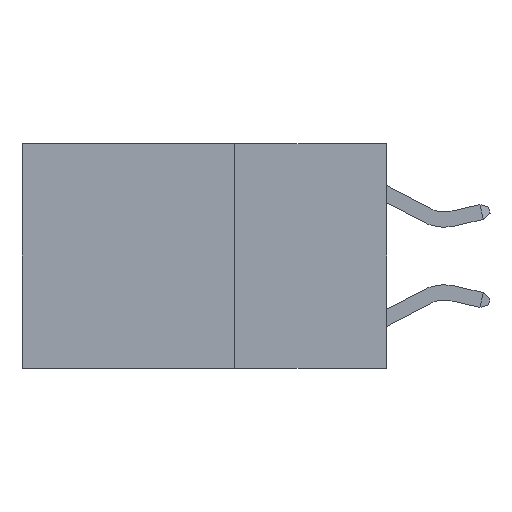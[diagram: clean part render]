
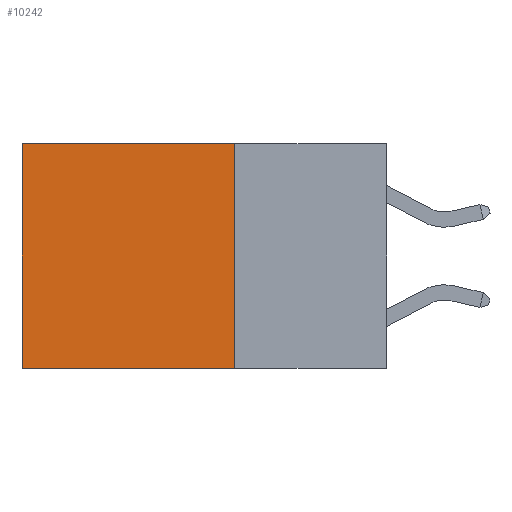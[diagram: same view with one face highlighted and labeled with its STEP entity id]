
A CAD part, left-side view. The second image highlights one B-rep face of the part: STEP entity #10242.
In plain terms, the highlighted planar face has unit normal (-1, 0, 0).
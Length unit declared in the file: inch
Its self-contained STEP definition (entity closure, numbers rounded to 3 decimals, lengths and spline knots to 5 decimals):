
#356 = DIRECTION ( 'NONE',  ( 0., 0., -1. ) ) ;
#781 = CARTESIAN_POINT ( 'NONE',  ( 0.2625, 0.25, -0.37 ) ) ;
#1396 = AXIS2_PLACEMENT_3D ( 'NONE', #16977, #13441, #356 ) ;
#1850 = LINE ( 'NONE', #19306, #15938 ) ;
#3019 = CARTESIAN_POINT ( 'NONE',  ( 0.2625, 0.25, -0.37 ) ) ;
#3358 = CARTESIAN_POINT ( 'NONE',  ( 0.2625, 0.6, -0.37 ) ) ;
#4898 = DIRECTION ( 'NONE',  ( 0., 0., -1. ) ) ;
#6145 = DIRECTION ( 'NONE',  ( 0., 0., -1. ) ) ;
#6592 = EDGE_CURVE ( 'NONE', #15354, #17855, #9353, .T. ) ;
#7827 = LINE ( 'NONE', #18238, #17997 ) ;
#9353 = LINE ( 'NONE', #781, #17417 ) ;
#9722 = CARTESIAN_POINT ( 'NONE',  ( 0.2625, 0.25, 0. ) ) ;
#9740 = CARTESIAN_POINT ( 'NONE',  ( 0.2625, 0.25, 0. ) ) ;
#9966 = DIRECTION ( 'NONE',  ( 0., 1., 0. ) ) ;
#10162 = EDGE_CURVE ( 'NONE', #11970, #15354, #7827, .T. ) ;
#10242 = ADVANCED_FACE ( 'NONE', ( #19570 ), #20124, .F. ) ;
#11108 = DIRECTION ( 'NONE',  ( 0., 1., 0. ) ) ;
#11970 = VERTEX_POINT ( 'NONE', #9722 ) ;
#12038 = ORIENTED_EDGE ( 'NONE', *, *, #6592, .F. ) ;
#13187 = LINE ( 'NONE', #9740, #18665 ) ;
#13441 = DIRECTION ( 'NONE',  ( 1., 0., 0. ) ) ;
#13506 = VERTEX_POINT ( 'NONE', #14209 ) ;
#14209 = CARTESIAN_POINT ( 'NONE',  ( 0.2625, 0.6, 0. ) ) ;
#14788 = ORIENTED_EDGE ( 'NONE', *, *, #18523, .T. ) ;
#15354 = VERTEX_POINT ( 'NONE', #3019 ) ;
#15938 = VECTOR ( 'NONE', #6145, 39.37008 ) ;
#16977 = CARTESIAN_POINT ( 'NONE',  ( 0.2625, 0.25, 0. ) ) ;
#17417 = VECTOR ( 'NONE', #11108, 39.37008 ) ;
#17855 = VERTEX_POINT ( 'NONE', #3358 ) ;
#17954 = ORIENTED_EDGE ( 'NONE', *, *, #10162, .F. ) ;
#17997 = VECTOR ( 'NONE', #4898, 39.37008 ) ;
#18238 = CARTESIAN_POINT ( 'NONE',  ( 0.2625, 0.25, 0. ) ) ;
#18523 = EDGE_CURVE ( 'NONE', #11970, #13506, #13187, .T. ) ;
#18665 = VECTOR ( 'NONE', #9966, 39.37008 ) ;
#19279 = EDGE_LOOP ( 'NONE', ( #19480, #12038, #17954, #14788 ) ) ;
#19306 = CARTESIAN_POINT ( 'NONE',  ( 0.2625, 0.6, 0. ) ) ;
#19480 = ORIENTED_EDGE ( 'NONE', *, *, #21471, .T. ) ;
#19570 = FACE_OUTER_BOUND ( 'NONE', #19279, .T. ) ;
#20124 = PLANE ( 'NONE',  #1396 ) ;
#21471 = EDGE_CURVE ( 'NONE', #13506, #17855, #1850, .T. ) ;
